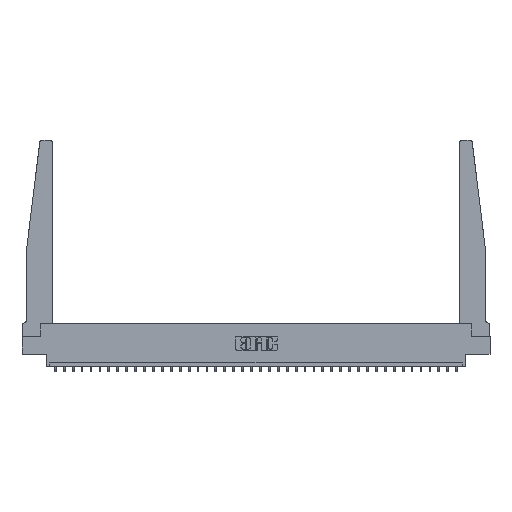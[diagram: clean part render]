
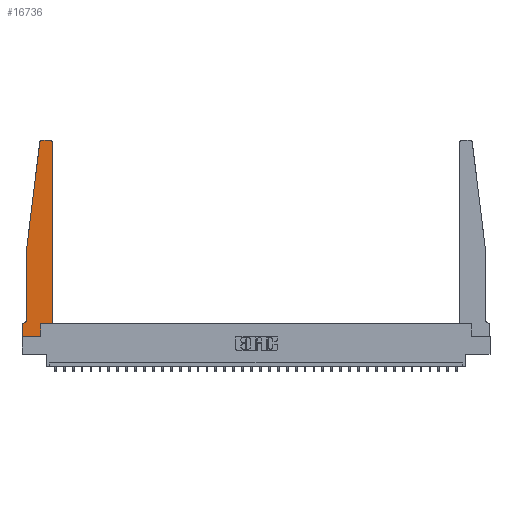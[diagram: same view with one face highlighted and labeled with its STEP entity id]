
A CAD part, top view. The second image highlights one B-rep face of the part: STEP entity #16736.
In plain terms, the highlighted planar face has unit normal (0, 0, 1).
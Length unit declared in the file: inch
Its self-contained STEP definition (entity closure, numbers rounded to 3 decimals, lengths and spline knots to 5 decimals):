
#68 = CARTESIAN_POINT ( 'NONE',  ( 0.065, 0.1875, 0.37 ) ) ;
#103 = LINE ( 'NONE', #23447, #9597 ) ;
#264 = DIRECTION ( 'NONE',  ( 1., 0., 0. ) ) ;
#672 = CARTESIAN_POINT ( 'NONE',  ( 0.395, 2.75, 0.37 ) ) ;
#882 = DIRECTION ( 'NONE',  ( 0., 0., 1. ) ) ;
#1530 = VERTEX_POINT ( 'NONE', #1733 ) ;
#1733 = CARTESIAN_POINT ( 'NONE',  ( 0.27653, 2.75, 0.37 ) ) ;
#1734 = DIRECTION ( 'NONE',  ( -0.122, -0.992, 0. ) ) ;
#2174 = ORIENTED_EDGE ( 'NONE', *, *, #7340, .T. ) ;
#2624 = DIRECTION ( 'NONE',  ( -1., 0., 0. ) ) ;
#3436 = CARTESIAN_POINT ( 'NONE',  ( 0., 0.1875, 0.37 ) ) ;
#3445 = CARTESIAN_POINT ( 'NONE',  ( 0.425, 0.18, 0.37 ) ) ;
#3609 = AXIS2_PLACEMENT_3D ( 'NONE', #9397, #19709, #30012 ) ;
#3624 = EDGE_CURVE ( 'NONE', #9303, #16000, #27713, .T. ) ;
#3646 = LINE ( 'NONE', #14301, #28504 ) ;
#3965 = VERTEX_POINT ( 'NONE', #20289 ) ;
#4107 = DIRECTION ( 'NONE',  ( 1., 0., 0. ) ) ;
#4113 = LINE ( 'NONE', #14611, #31066 ) ;
#5191 = AXIS2_PLACEMENT_3D ( 'NONE', #3436, #882, #4107 ) ;
#5302 = VERTEX_POINT ( 'NONE', #7763 ) ;
#5864 = ORIENTED_EDGE ( 'NONE', *, *, #27604, .T. ) ;
#6374 = EDGE_CURVE ( 'NONE', #5302, #3965, #4113, .T. ) ;
#6844 = ORIENTED_EDGE ( 'NONE', *, *, #23477, .T. ) ;
#7340 = EDGE_CURVE ( 'NONE', #33072, #25556, #7699, .T. ) ;
#7591 = VERTEX_POINT ( 'NONE', #3445 ) ;
#7699 = LINE ( 'NONE', #68, #28940 ) ;
#7763 = CARTESIAN_POINT ( 'NONE',  ( 0.24675, 2.72367, 0.37 ) ) ;
#8073 = DIRECTION ( 'NONE',  ( 0., 0., 1. ) ) ;
#8750 = VERTEX_POINT ( 'NONE', #25532 ) ;
#8922 = CARTESIAN_POINT ( 'NONE',  ( 0.25, 2.75, 0.37 ) ) ;
#9303 = VERTEX_POINT ( 'NONE', #31385 ) ;
#9397 = CARTESIAN_POINT ( 'NONE',  ( 0.015, 0.2375, 0.37 ) ) ;
#9516 = EDGE_CURVE ( 'NONE', #16000, #7591, #3646, .T. ) ;
#9597 = VECTOR ( 'NONE', #264, 39.37008 ) ;
#9855 = DIRECTION ( 'NONE',  ( 0., -1., 0. ) ) ;
#10615 = CARTESIAN_POINT ( 'NONE',  ( 0.395, 2.72, 0.37 ) ) ;
#10933 = VECTOR ( 'NONE', #26211, 39.37008 ) ;
#11256 = EDGE_CURVE ( 'NONE', #3965, #19398, #14109, .T. ) ;
#12380 = AXIS2_PLACEMENT_3D ( 'NONE', #10615, #8073, #18397 ) ;
#12949 = ORIENTED_EDGE ( 'NONE', *, *, #27255, .T. ) ;
#13719 = EDGE_LOOP ( 'NONE', ( #25930, #6844, #13924, #19473, #25599, #2174, #12949, #29834, #22002, #31162, #5864, #30172 ) ) ;
#13924 = ORIENTED_EDGE ( 'NONE', *, *, #6374, .T. ) ;
#14109 = LINE ( 'NONE', #24413, #22102 ) ;
#14301 = CARTESIAN_POINT ( 'NONE',  ( 0.425, 0.18, 0.37 ) ) ;
#14611 = CARTESIAN_POINT ( 'NONE',  ( 0.065, 1.25, 0.37 ) ) ;
#14648 = DIRECTION ( 'NONE',  ( 1., 0., 0. ) ) ;
#14830 = CARTESIAN_POINT ( 'NONE',  ( 0.065, 0.2375, 0.37 ) ) ;
#15087 = LINE ( 'NONE', #27598, #22269 ) ;
#15189 = VERTEX_POINT ( 'NONE', #672 ) ;
#15945 = VECTOR ( 'NONE', #31903, 39.37008 ) ;
#16000 = VERTEX_POINT ( 'NONE', #27891 ) ;
#16413 = LINE ( 'NONE', #31451, #10933 ) ;
#16698 = CIRCLE ( 'NONE', #12380, 0.03 ) ;
#16736 = ADVANCED_FACE ( 'NONE', ( #26604 ), #22028, .T. ) ;
#18397 = DIRECTION ( 'NONE',  ( 1., 0., 0. ) ) ;
#18728 = CIRCLE ( 'NONE', #3609, 0.05 ) ;
#18736 = LINE ( 'NONE', #8922, #15945 ) ;
#19398 = VERTEX_POINT ( 'NONE', #14830 ) ;
#19473 = ORIENTED_EDGE ( 'NONE', *, *, #11256, .T. ) ;
#19709 = DIRECTION ( 'NONE',  ( 0., 0., -1. ) ) ;
#20193 = EDGE_CURVE ( 'NONE', #30714, #9303, #103, .T. ) ;
#20289 = CARTESIAN_POINT ( 'NONE',  ( 0.065, 1.25, 0.37 ) ) ;
#21019 = DIRECTION ( 'NONE',  ( 0., 0., 1. ) ) ;
#21424 = EDGE_CURVE ( 'NONE', #8750, #15189, #16698, .T. ) ;
#22002 = ORIENTED_EDGE ( 'NONE', *, *, #3624, .T. ) ;
#22028 = PLANE ( 'NONE',  #5191 ) ;
#22102 = VECTOR ( 'NONE', #24923, 39.37008 ) ;
#22269 = VECTOR ( 'NONE', #9855, 39.37008 ) ;
#23244 = CIRCLE ( 'NONE', #27569, 0.03 ) ;
#23447 = CARTESIAN_POINT ( 'NONE',  ( 0., 0., 0.37 ) ) ;
#23471 = VECTOR ( 'NONE', #32944, 39.37008 ) ;
#23477 = EDGE_CURVE ( 'NONE', #1530, #5302, #23244, .T. ) ;
#24413 = CARTESIAN_POINT ( 'NONE',  ( 0.065, 1.25, 0.37 ) ) ;
#24923 = DIRECTION ( 'NONE',  ( 0., -1., 0. ) ) ;
#25350 = CARTESIAN_POINT ( 'NONE',  ( 0.2605, 0.18, 0.37 ) ) ;
#25532 = CARTESIAN_POINT ( 'NONE',  ( 0.425, 2.72, 0.37 ) ) ;
#25556 = VERTEX_POINT ( 'NONE', #32348 ) ;
#25599 = ORIENTED_EDGE ( 'NONE', *, *, #32267, .T. ) ;
#25770 = CARTESIAN_POINT ( 'NONE',  ( 0., 0., 0.37 ) ) ;
#25930 = ORIENTED_EDGE ( 'NONE', *, *, #28508, .T. ) ;
#26211 = DIRECTION ( 'NONE',  ( 0., 1., 0. ) ) ;
#26604 = FACE_OUTER_BOUND ( 'NONE', #13719, .T. ) ;
#27255 = EDGE_CURVE ( 'NONE', #25556, #30714, #15087, .T. ) ;
#27401 = CARTESIAN_POINT ( 'NONE',  ( 0.015, 0.1875, 0.37 ) ) ;
#27569 = AXIS2_PLACEMENT_3D ( 'NONE', #27958, #21019, #30662 ) ;
#27598 = CARTESIAN_POINT ( 'NONE',  ( 0., 0., 0.37 ) ) ;
#27604 = EDGE_CURVE ( 'NONE', #7591, #8750, #16413, .T. ) ;
#27713 = LINE ( 'NONE', #25350, #23471 ) ;
#27891 = CARTESIAN_POINT ( 'NONE',  ( 0.2605, 0.18, 0.37 ) ) ;
#27958 = CARTESIAN_POINT ( 'NONE',  ( 0.27653, 2.72, 0.37 ) ) ;
#28504 = VECTOR ( 'NONE', #14648, 39.37008 ) ;
#28508 = EDGE_CURVE ( 'NONE', #15189, #1530, #18736, .T. ) ;
#28940 = VECTOR ( 'NONE', #2624, 39.37008 ) ;
#29834 = ORIENTED_EDGE ( 'NONE', *, *, #20193, .T. ) ;
#30012 = DIRECTION ( 'NONE',  ( -1., 0., 0. ) ) ;
#30172 = ORIENTED_EDGE ( 'NONE', *, *, #21424, .T. ) ;
#30662 = DIRECTION ( 'NONE',  ( 1., 0., 0. ) ) ;
#30714 = VERTEX_POINT ( 'NONE', #25770 ) ;
#31066 = VECTOR ( 'NONE', #1734, 39.37008 ) ;
#31162 = ORIENTED_EDGE ( 'NONE', *, *, #9516, .T. ) ;
#31385 = CARTESIAN_POINT ( 'NONE',  ( 0.2605, 0., 0.37 ) ) ;
#31451 = CARTESIAN_POINT ( 'NONE',  ( 0.425, 0.18, 0.37 ) ) ;
#31903 = DIRECTION ( 'NONE',  ( -1., 0., 0. ) ) ;
#32267 = EDGE_CURVE ( 'NONE', #19398, #33072, #18728, .T. ) ;
#32348 = CARTESIAN_POINT ( 'NONE',  ( 0., 0.1875, 0.37 ) ) ;
#32944 = DIRECTION ( 'NONE',  ( 0., 1., 0. ) ) ;
#33072 = VERTEX_POINT ( 'NONE', #27401 ) ;
